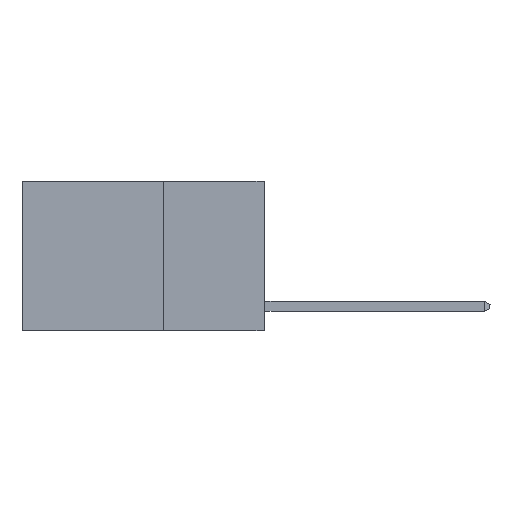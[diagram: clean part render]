
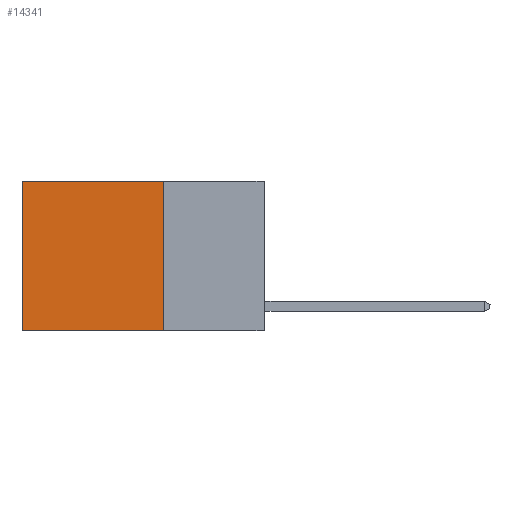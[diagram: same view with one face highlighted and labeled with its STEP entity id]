
A CAD part, left-side view. The second image highlights one B-rep face of the part: STEP entity #14341.
In plain terms, the highlighted planar face has unit normal (-1, 0, 0).
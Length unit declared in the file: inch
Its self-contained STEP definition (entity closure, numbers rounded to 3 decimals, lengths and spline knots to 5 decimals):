
#27 = PLANE ( 'NONE',  #11729 ) ;
#102 = EDGE_CURVE ( 'NONE', #10643, #17471, #11889, .T. ) ;
#993 = CARTESIAN_POINT ( 'NONE',  ( 0.2625, 0.6, 0. ) ) ;
#1895 = EDGE_LOOP ( 'NONE', ( #15416, #3791, #4419, #3175 ) ) ;
#2050 = CARTESIAN_POINT ( 'NONE',  ( 0.2625, 0.25, 0. ) ) ;
#2531 = CARTESIAN_POINT ( 'NONE',  ( 0.2625, 0.25, 0. ) ) ;
#3175 = ORIENTED_EDGE ( 'NONE', *, *, #9852, .T. ) ;
#3791 = ORIENTED_EDGE ( 'NONE', *, *, #102, .F. ) ;
#4384 = DIRECTION ( 'NONE',  ( 1., 0., 0. ) ) ;
#4419 = ORIENTED_EDGE ( 'NONE', *, *, #9293, .F. ) ;
#5815 = VECTOR ( 'NONE', #16272, 39.37008 ) ;
#6003 = VECTOR ( 'NONE', #10867, 39.37008 ) ;
#6370 = CARTESIAN_POINT ( 'NONE',  ( 0.2625, 0.25, 0. ) ) ;
#6962 = DIRECTION ( 'NONE',  ( 0., 0., -1. ) ) ;
#6996 = VECTOR ( 'NONE', #11195, 39.37008 ) ;
#7082 = CARTESIAN_POINT ( 'NONE',  ( 0.2625, 0.25, -0.37 ) ) ;
#7332 = LINE ( 'NONE', #993, #6003 ) ;
#7501 = DIRECTION ( 'NONE',  ( 0., 0., -1. ) ) ;
#8577 = CARTESIAN_POINT ( 'NONE',  ( 0.2625, 0.6, -0.37 ) ) ;
#9293 = EDGE_CURVE ( 'NONE', #16463, #10643, #14693, .T. ) ;
#9591 = CARTESIAN_POINT ( 'NONE',  ( 0.2625, 0.25, -0.37 ) ) ;
#9852 = EDGE_CURVE ( 'NONE', #16463, #13316, #14213, .T. ) ;
#10643 = VERTEX_POINT ( 'NONE', #7082 ) ;
#10867 = DIRECTION ( 'NONE',  ( 0., 0., -1. ) ) ;
#10906 = VECTOR ( 'NONE', #6962, 39.37008 ) ;
#11075 = CARTESIAN_POINT ( 'NONE',  ( 0.2625, 0.6, 0. ) ) ;
#11195 = DIRECTION ( 'NONE',  ( 0., 1., 0. ) ) ;
#11729 = AXIS2_PLACEMENT_3D ( 'NONE', #13861, #4384, #7501 ) ;
#11889 = LINE ( 'NONE', #9591, #6996 ) ;
#13316 = VERTEX_POINT ( 'NONE', #11075 ) ;
#13861 = CARTESIAN_POINT ( 'NONE',  ( 0.2625, 0.25, 0. ) ) ;
#14213 = LINE ( 'NONE', #2050, #5815 ) ;
#14341 = ADVANCED_FACE ( 'NONE', ( #15519 ), #27, .F. ) ;
#14380 = EDGE_CURVE ( 'NONE', #13316, #17471, #7332, .T. ) ;
#14693 = LINE ( 'NONE', #2531, #10906 ) ;
#15416 = ORIENTED_EDGE ( 'NONE', *, *, #14380, .T. ) ;
#15519 = FACE_OUTER_BOUND ( 'NONE', #1895, .T. ) ;
#16272 = DIRECTION ( 'NONE',  ( 0., 1., 0. ) ) ;
#16463 = VERTEX_POINT ( 'NONE', #6370 ) ;
#17471 = VERTEX_POINT ( 'NONE', #8577 ) ;
